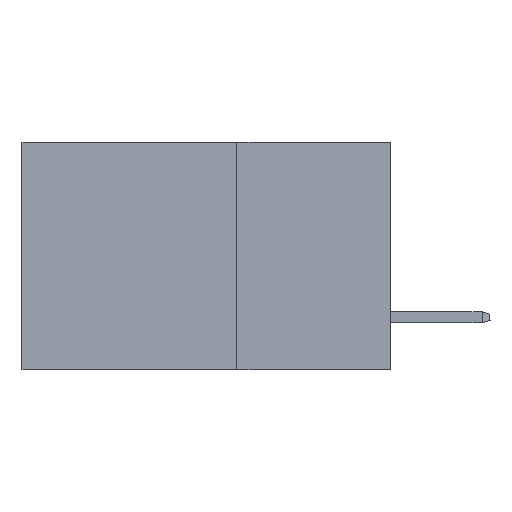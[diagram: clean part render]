
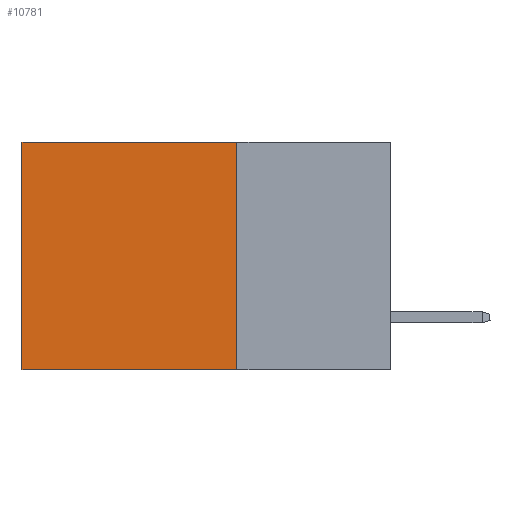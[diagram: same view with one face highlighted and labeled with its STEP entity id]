
A CAD part, left-side view. The second image highlights one B-rep face of the part: STEP entity #10781.
In plain terms, the highlighted planar face has unit normal (-1, 0, 0).
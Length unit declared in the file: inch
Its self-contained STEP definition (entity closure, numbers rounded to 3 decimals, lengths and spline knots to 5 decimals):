
#331 = ORIENTED_EDGE ( 'NONE', *, *, #13586, .F. ) ;
#1217 = EDGE_LOOP ( 'NONE', ( #9004, #20395, #331, #16912 ) ) ;
#2485 = CARTESIAN_POINT ( 'NONE',  ( 0.2875, 0.25, 0. ) ) ;
#3143 = VECTOR ( 'NONE', #18990, 39.37008 ) ;
#5870 = CARTESIAN_POINT ( 'NONE',  ( 0.2875, 0.25, 0. ) ) ;
#6935 = CARTESIAN_POINT ( 'NONE',  ( 0.2875, 0.25, -0.37 ) ) ;
#7866 = VERTEX_POINT ( 'NONE', #12706 ) ;
#9004 = ORIENTED_EDGE ( 'NONE', *, *, #14817, .T. ) ;
#10517 = VECTOR ( 'NONE', #13128, 39.37008 ) ;
#10781 = ADVANCED_FACE ( 'NONE', ( #27281 ), #25918, .F. ) ;
#11198 = EDGE_CURVE ( 'NONE', #27258, #20778, #14146, .T. ) ;
#11427 = AXIS2_PLACEMENT_3D ( 'NONE', #26385, #13596, #19997 ) ;
#12593 = LINE ( 'NONE', #25201, #3143 ) ;
#12706 = CARTESIAN_POINT ( 'NONE',  ( 0.2875, 0.6, 0. ) ) ;
#13128 = DIRECTION ( 'NONE',  ( 0., 0., -1. ) ) ;
#13327 = CARTESIAN_POINT ( 'NONE',  ( 0.2875, 0.6, 0. ) ) ;
#13586 = EDGE_CURVE ( 'NONE', #20008, #27258, #12593, .T. ) ;
#13596 = DIRECTION ( 'NONE',  ( 1., 0., 0. ) ) ;
#14146 = LINE ( 'NONE', #17493, #19174 ) ;
#14817 = EDGE_CURVE ( 'NONE', #7866, #20778, #17257, .T. ) ;
#16912 = ORIENTED_EDGE ( 'NONE', *, *, #24895, .T. ) ;
#17038 = LINE ( 'NONE', #5870, #19731 ) ;
#17257 = LINE ( 'NONE', #13327, #10517 ) ;
#17493 = CARTESIAN_POINT ( 'NONE',  ( 0.2875, 0.25, -0.37 ) ) ;
#18990 = DIRECTION ( 'NONE',  ( 0., 0., -1. ) ) ;
#19174 = VECTOR ( 'NONE', #21534, 39.37008 ) ;
#19731 = VECTOR ( 'NONE', #23621, 39.37008 ) ;
#19997 = DIRECTION ( 'NONE',  ( 0., 0., -1. ) ) ;
#20008 = VERTEX_POINT ( 'NONE', #2485 ) ;
#20395 = ORIENTED_EDGE ( 'NONE', *, *, #11198, .F. ) ;
#20778 = VERTEX_POINT ( 'NONE', #26973 ) ;
#21534 = DIRECTION ( 'NONE',  ( 0., 1., 0. ) ) ;
#23621 = DIRECTION ( 'NONE',  ( 0., 1., 0. ) ) ;
#24895 = EDGE_CURVE ( 'NONE', #20008, #7866, #17038, .T. ) ;
#25201 = CARTESIAN_POINT ( 'NONE',  ( 0.2875, 0.25, 0. ) ) ;
#25918 = PLANE ( 'NONE',  #11427 ) ;
#26385 = CARTESIAN_POINT ( 'NONE',  ( 0.2875, 0.25, 0. ) ) ;
#26973 = CARTESIAN_POINT ( 'NONE',  ( 0.2875, 0.6, -0.37 ) ) ;
#27258 = VERTEX_POINT ( 'NONE', #6935 ) ;
#27281 = FACE_OUTER_BOUND ( 'NONE', #1217, .T. ) ;
